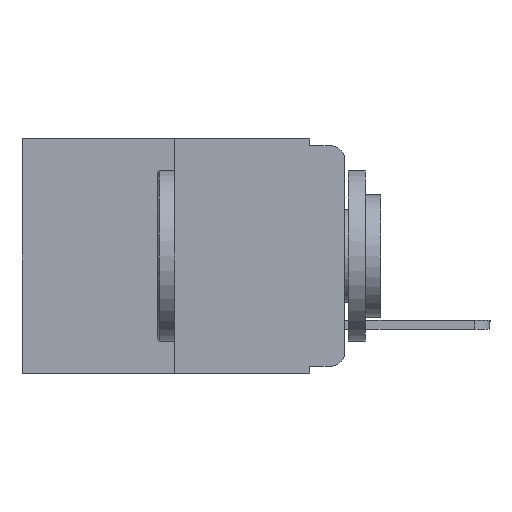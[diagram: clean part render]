
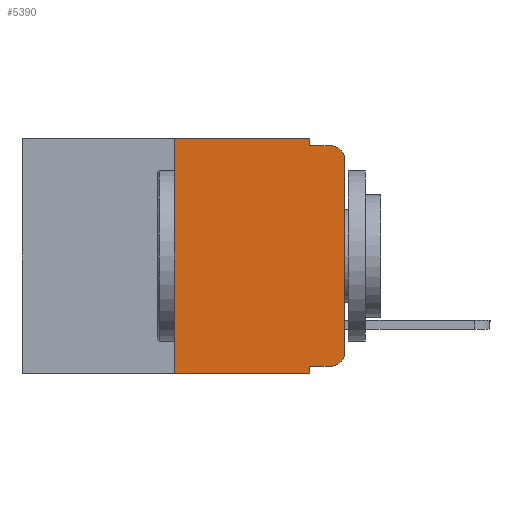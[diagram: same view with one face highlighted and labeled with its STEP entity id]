
A CAD part, left-side view. The second image highlights one B-rep face of the part: STEP entity #5390.
In plain terms, the highlighted planar face has unit normal (-1, 0, 0).
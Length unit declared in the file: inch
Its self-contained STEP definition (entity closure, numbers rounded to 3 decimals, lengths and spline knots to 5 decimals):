
#37 = CARTESIAN_POINT ( 'NONE',  ( 0., 0.25, -0.343 ) ) ;
#142 = VERTEX_POINT ( 'NONE', #19650 ) ;
#228 = DIRECTION ( 'NONE',  ( 0., 0., -1. ) ) ;
#327 = VERTEX_POINT ( 'NONE', #3398 ) ;
#458 = CARTESIAN_POINT ( 'NONE',  ( 0., 0.051, 0. ) ) ;
#535 = DIRECTION ( 'NONE',  ( 1., 0., 0. ) ) ;
#1643 = VECTOR ( 'NONE', #7703, 39.37008 ) ;
#1875 = CARTESIAN_POINT ( 'NONE',  ( 0., 0.473, -0.343 ) ) ;
#2317 = VECTOR ( 'NONE', #16470, 39.37008 ) ;
#2673 = VECTOR ( 'NONE', #10971, 39.37008 ) ;
#2736 = CARTESIAN_POINT ( 'NONE',  ( 0., 0.051, -0.01 ) ) ;
#2911 = CARTESIAN_POINT ( 'NONE',  ( 0., 0.051, -0.333 ) ) ;
#3006 = VECTOR ( 'NONE', #17581, 39.37008 ) ;
#3324 = CARTESIAN_POINT ( 'NONE',  ( 0., 0.051, 0. ) ) ;
#3333 = VECTOR ( 'NONE', #17488, 39.37008 ) ;
#3398 = CARTESIAN_POINT ( 'NONE',  ( 0., 0., -0.313 ) ) ;
#3463 = ORIENTED_EDGE ( 'NONE', *, *, #7638, .F. ) ;
#3478 = EDGE_CURVE ( 'NONE', #6777, #327, #7219, .T. ) ;
#3542 = CARTESIAN_POINT ( 'NONE',  ( 0., 0.473, 0. ) ) ;
#3609 = LINE ( 'NONE', #1875, #3006 ) ;
#3881 = ORIENTED_EDGE ( 'NONE', *, *, #4089, .T. ) ;
#4089 = EDGE_CURVE ( 'NONE', #19621, #8199, #3609, .T. ) ;
#4194 = LINE ( 'NONE', #10421, #7912 ) ;
#4312 = CARTESIAN_POINT ( 'NONE',  ( 0., 0., -0.03 ) ) ;
#4373 = DIRECTION ( 'NONE',  ( -1., 0., 0. ) ) ;
#4518 = ORIENTED_EDGE ( 'NONE', *, *, #3478, .T. ) ;
#4689 = DIRECTION ( 'NONE',  ( 0., -1., 0. ) ) ;
#4840 = LINE ( 'NONE', #6587, #3333 ) ;
#4880 = ORIENTED_EDGE ( 'NONE', *, *, #14210, .F. ) ;
#5017 = VERTEX_POINT ( 'NONE', #458 ) ;
#5065 = VERTEX_POINT ( 'NONE', #12701 ) ;
#5390 = ADVANCED_FACE ( 'NONE', ( #14227 ), #6578, .F. ) ;
#6252 = AXIS2_PLACEMENT_3D ( 'NONE', #17102, #4373, #13951 ) ;
#6418 = ORIENTED_EDGE ( 'NONE', *, *, #17220, .F. ) ;
#6578 = PLANE ( 'NONE',  #18614 ) ;
#6587 = CARTESIAN_POINT ( 'NONE',  ( 0., 0.051, -0.01 ) ) ;
#6714 = VERTEX_POINT ( 'NONE', #4312 ) ;
#6777 = VERTEX_POINT ( 'NONE', #19803 ) ;
#7219 = CIRCLE ( 'NONE', #6252, 0.02 ) ;
#7230 = EDGE_LOOP ( 'NONE', ( #19433, #7331, #4880, #3463, #15431, #15719, #3881, #6418, #9628, #4518 ) ) ;
#7331 = ORIENTED_EDGE ( 'NONE', *, *, #13510, .T. ) ;
#7638 = EDGE_CURVE ( 'NONE', #5017, #17141, #19934, .T. ) ;
#7703 = DIRECTION ( 'NONE',  ( 0., -1., 0. ) ) ;
#7912 = VECTOR ( 'NONE', #16644, 39.37008 ) ;
#8199 = VERTEX_POINT ( 'NONE', #12545 ) ;
#9628 = ORIENTED_EDGE ( 'NONE', *, *, #12568, .T. ) ;
#10249 = CARTESIAN_POINT ( 'NONE',  ( 0., 0.051, 0. ) ) ;
#10392 = CARTESIAN_POINT ( 'NONE',  ( 0., 0.25, 0. ) ) ;
#10421 = CARTESIAN_POINT ( 'NONE',  ( 0., 0.25, 0. ) ) ;
#10971 = DIRECTION ( 'NONE',  ( 0., 0., -1. ) ) ;
#11177 = LINE ( 'NONE', #3324, #2673 ) ;
#12545 = CARTESIAN_POINT ( 'NONE',  ( 0., 0.051, -0.343 ) ) ;
#12568 = EDGE_CURVE ( 'NONE', #142, #6777, #15452, .T. ) ;
#12621 = LINE ( 'NONE', #3542, #19877 ) ;
#12701 = CARTESIAN_POINT ( 'NONE',  ( 0., 0.02, -0.01 ) ) ;
#13510 = EDGE_CURVE ( 'NONE', #6714, #5065, #19598, .T. ) ;
#13951 = DIRECTION ( 'NONE',  ( 0., 0., -1. ) ) ;
#14210 = EDGE_CURVE ( 'NONE', #17141, #5065, #4840, .T. ) ;
#14227 = FACE_OUTER_BOUND ( 'NONE', #7230, .T. ) ;
#14441 = CARTESIAN_POINT ( 'NONE',  ( 0., 0.473, 0. ) ) ;
#14716 = LINE ( 'NONE', #17770, #18611 ) ;
#15068 = CARTESIAN_POINT ( 'NONE',  ( 0., 0.02, -0.03 ) ) ;
#15431 = ORIENTED_EDGE ( 'NONE', *, *, #16857, .F. ) ;
#15452 = LINE ( 'NONE', #2911, #1643 ) ;
#15719 = ORIENTED_EDGE ( 'NONE', *, *, #19843, .F. ) ;
#16342 = AXIS2_PLACEMENT_3D ( 'NONE', #15068, #18024, #19449 ) ;
#16470 = DIRECTION ( 'NONE',  ( 0., 0., -1. ) ) ;
#16644 = DIRECTION ( 'NONE',  ( 0., 0., 1. ) ) ;
#16857 = EDGE_CURVE ( 'NONE', #19048, #5017, #12621, .T. ) ;
#17102 = CARTESIAN_POINT ( 'NONE',  ( 0., 0.02, -0.313 ) ) ;
#17141 = VERTEX_POINT ( 'NONE', #2736 ) ;
#17220 = EDGE_CURVE ( 'NONE', #142, #8199, #11177, .T. ) ;
#17488 = DIRECTION ( 'NONE',  ( 0., -1., 0. ) ) ;
#17581 = DIRECTION ( 'NONE',  ( 0., -1., 0. ) ) ;
#17770 = CARTESIAN_POINT ( 'NONE',  ( 0., 0., 0. ) ) ;
#18024 = DIRECTION ( 'NONE',  ( -1., 0., 0. ) ) ;
#18513 = EDGE_CURVE ( 'NONE', #327, #6714, #14716, .T. ) ;
#18611 = VECTOR ( 'NONE', #19498, 39.37008 ) ;
#18614 = AXIS2_PLACEMENT_3D ( 'NONE', #14441, #535, #228 ) ;
#19048 = VERTEX_POINT ( 'NONE', #10392 ) ;
#19433 = ORIENTED_EDGE ( 'NONE', *, *, #18513, .T. ) ;
#19449 = DIRECTION ( 'NONE',  ( 0., 0., -1. ) ) ;
#19498 = DIRECTION ( 'NONE',  ( 0., 0., 1. ) ) ;
#19598 = CIRCLE ( 'NONE', #16342, 0.02 ) ;
#19621 = VERTEX_POINT ( 'NONE', #37 ) ;
#19650 = CARTESIAN_POINT ( 'NONE',  ( 0., 0.051, -0.333 ) ) ;
#19803 = CARTESIAN_POINT ( 'NONE',  ( 0., 0.02, -0.333 ) ) ;
#19843 = EDGE_CURVE ( 'NONE', #19621, #19048, #4194, .T. ) ;
#19877 = VECTOR ( 'NONE', #4689, 39.37008 ) ;
#19934 = LINE ( 'NONE', #10249, #2317 ) ;
